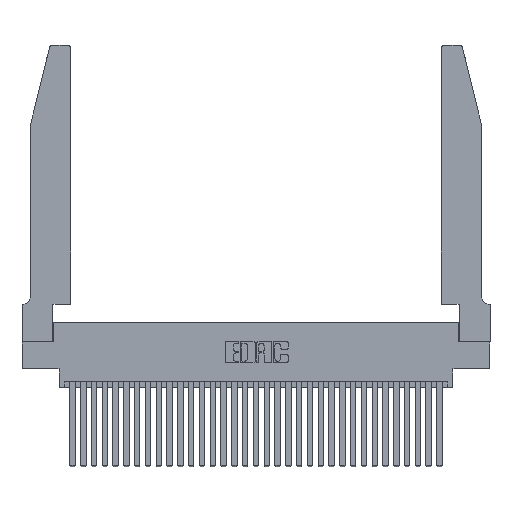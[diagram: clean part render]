
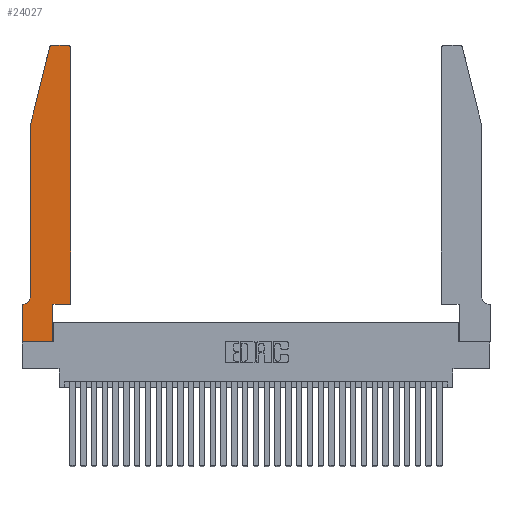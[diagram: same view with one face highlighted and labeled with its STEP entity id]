
A CAD part, top view. The second image highlights one B-rep face of the part: STEP entity #24027.
In plain terms, the highlighted planar face has unit normal (0, 0, 1).
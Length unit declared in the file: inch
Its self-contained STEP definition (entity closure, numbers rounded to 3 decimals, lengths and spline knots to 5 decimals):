
#411 = AXIS2_PLACEMENT_3D ( 'NONE', #13067, #10168, #25579 ) ;
#999 = CARTESIAN_POINT ( 'NONE',  ( 0.0755, 2., 0.37 ) ) ;
#1209 = CARTESIAN_POINT ( 'NONE',  ( 0.4505, 2.72, 0.37 ) ) ;
#1356 = LINE ( 'NONE', #23913, #9742 ) ;
#1509 = DIRECTION ( 'NONE',  ( -1., 0., 0. ) ) ;
#1685 = CARTESIAN_POINT ( 'NONE',  ( 0.2865, 0., 0.37 ) ) ;
#1832 = EDGE_CURVE ( 'NONE', #4338, #18854, #30496, .T. ) ;
#1875 = VERTEX_POINT ( 'NONE', #2177 ) ;
#1903 = LINE ( 'NONE', #19089, #4674 ) ;
#1988 = AXIS2_PLACEMENT_3D ( 'NONE', #17093, #2187, #29643 ) ;
#2177 = CARTESIAN_POINT ( 'NONE',  ( 0.284, 2.75, 0.37 ) ) ;
#2187 = DIRECTION ( 'NONE',  ( 0., 0., 1. ) ) ;
#2234 = LINE ( 'NONE', #25883, #6675 ) ;
#2886 = DIRECTION ( 'NONE',  ( 1., 0., 0. ) ) ;
#3325 = ORIENTED_EDGE ( 'NONE', *, *, #1832, .T. ) ;
#3663 = LINE ( 'NONE', #13820, #12471 ) ;
#3780 = DIRECTION ( 'NONE',  ( 0., -1., 0. ) ) ;
#3794 = ORIENTED_EDGE ( 'NONE', *, *, #19834, .T. ) ;
#4338 = VERTEX_POINT ( 'NONE', #27842 ) ;
#4674 = VECTOR ( 'NONE', #3780, 39.37008 ) ;
#5346 = PLANE ( 'NONE',  #411 ) ;
#5381 = VERTEX_POINT ( 'NONE', #8196 ) ;
#6237 = CIRCLE ( 'NONE', #1988, 0.03 ) ;
#6628 = FACE_OUTER_BOUND ( 'NONE', #9629, .T. ) ;
#6675 = VECTOR ( 'NONE', #2886, 39.37008 ) ;
#7281 = CIRCLE ( 'NONE', #28473, 0.03 ) ;
#7554 = DIRECTION ( 'NONE',  ( 0., 0., 1. ) ) ;
#7750 = ORIENTED_EDGE ( 'NONE', *, *, #16142, .T. ) ;
#8196 = CARTESIAN_POINT ( 'NONE',  ( 0.4205, 2.75, 0.37 ) ) ;
#8215 = ORIENTED_EDGE ( 'NONE', *, *, #14040, .T. ) ;
#8622 = ORIENTED_EDGE ( 'NONE', *, *, #14255, .T. ) ;
#9404 = CARTESIAN_POINT ( 'NONE',  ( 0., 0., 0.37 ) ) ;
#9629 = EDGE_LOOP ( 'NONE', ( #24375, #29802, #29660, #8622, #3325, #3794, #8215, #16254, #21913, #7750, #10709, #12995 ) ) ;
#9638 = VERTEX_POINT ( 'NONE', #17158 ) ;
#9742 = VECTOR ( 'NONE', #19107, 39.37008 ) ;
#10168 = DIRECTION ( 'NONE',  ( 0., 0., 1. ) ) ;
#10709 = ORIENTED_EDGE ( 'NONE', *, *, #17908, .T. ) ;
#12313 = AXIS2_PLACEMENT_3D ( 'NONE', #17534, #12477, #25004 ) ;
#12471 = VECTOR ( 'NONE', #29265, 39.37008 ) ;
#12477 = DIRECTION ( 'NONE',  ( 0., 0., -1. ) ) ;
#12713 = CARTESIAN_POINT ( 'NONE',  ( 0.2865, 0.35, 0.37 ) ) ;
#12995 = ORIENTED_EDGE ( 'NONE', *, *, #32623, .T. ) ;
#13067 = CARTESIAN_POINT ( 'NONE',  ( 0., 0.35, 0.37 ) ) ;
#13820 = CARTESIAN_POINT ( 'NONE',  ( 0.2605, 2.75, 0.37 ) ) ;
#14040 = EDGE_CURVE ( 'NONE', #9638, #29426, #1903, .T. ) ;
#14255 = EDGE_CURVE ( 'NONE', #29400, #4338, #18671, .T. ) ;
#14325 = DIRECTION ( 'NONE',  ( 1., 0., 0. ) ) ;
#14371 = VERTEX_POINT ( 'NONE', #19503 ) ;
#14756 = LINE ( 'NONE', #20382, #18322 ) ;
#14765 = CARTESIAN_POINT ( 'NONE',  ( 0.0755, 2., 0.37 ) ) ;
#15058 = EDGE_CURVE ( 'NONE', #1875, #17614, #6237, .T. ) ;
#15329 = LINE ( 'NONE', #24484, #25692 ) ;
#16114 = CARTESIAN_POINT ( 'NONE',  ( 0.4505, 0.35, 0.37 ) ) ;
#16142 = EDGE_CURVE ( 'NONE', #19496, #14371, #2234, .T. ) ;
#16254 = ORIENTED_EDGE ( 'NONE', *, *, #24840, .T. ) ;
#17093 = CARTESIAN_POINT ( 'NONE',  ( 0.284, 2.72, 0.37 ) ) ;
#17158 = CARTESIAN_POINT ( 'NONE',  ( 0., 0.35, 0.37 ) ) ;
#17427 = CARTESIAN_POINT ( 'NONE',  ( 0.4205, 2.72, 0.37 ) ) ;
#17497 = VECTOR ( 'NONE', #24241, 39.37008 ) ;
#17534 = CARTESIAN_POINT ( 'NONE',  ( 0.0055, 0.42, 0.37 ) ) ;
#17614 = VERTEX_POINT ( 'NONE', #29901 ) ;
#17908 = EDGE_CURVE ( 'NONE', #14371, #21235, #32936, .T. ) ;
#18322 = VECTOR ( 'NONE', #28211, 39.37008 ) ;
#18383 = DIRECTION ( 'NONE',  ( 0., 1., 0. ) ) ;
#18671 = LINE ( 'NONE', #999, #17497 ) ;
#18854 = VERTEX_POINT ( 'NONE', #30739 ) ;
#19089 = CARTESIAN_POINT ( 'NONE',  ( 0., 0., 0.37 ) ) ;
#19107 = DIRECTION ( 'NONE',  ( 0., 1., 0. ) ) ;
#19496 = VERTEX_POINT ( 'NONE', #12713 ) ;
#19503 = CARTESIAN_POINT ( 'NONE',  ( 0.4505, 0.35, 0.37 ) ) ;
#19834 = EDGE_CURVE ( 'NONE', #18854, #9638, #23213, .T. ) ;
#20352 = VERTEX_POINT ( 'NONE', #1685 ) ;
#20382 = CARTESIAN_POINT ( 'NONE',  ( 0.0755, 2., 0.37 ) ) ;
#21101 = EDGE_CURVE ( 'NONE', #17614, #29400, #14756, .T. ) ;
#21235 = VERTEX_POINT ( 'NONE', #1209 ) ;
#21913 = ORIENTED_EDGE ( 'NONE', *, *, #24751, .T. ) ;
#22615 = CARTESIAN_POINT ( 'NONE',  ( 0.0755, 0.35, 0.37 ) ) ;
#22852 = DIRECTION ( 'NONE',  ( 1., 0., 0. ) ) ;
#23213 = LINE ( 'NONE', #22615, #29267 ) ;
#23913 = CARTESIAN_POINT ( 'NONE',  ( 0.2865, 0.35, 0.37 ) ) ;
#24027 = ADVANCED_FACE ( 'NONE', ( #6628 ), #5346, .T. ) ;
#24241 = DIRECTION ( 'NONE',  ( 0., -1., 0. ) ) ;
#24375 = ORIENTED_EDGE ( 'NONE', *, *, #32944, .T. ) ;
#24484 = CARTESIAN_POINT ( 'NONE',  ( 0., 0., 0.37 ) ) ;
#24751 = EDGE_CURVE ( 'NONE', #20352, #19496, #1356, .T. ) ;
#24840 = EDGE_CURVE ( 'NONE', #29426, #20352, #15329, .T. ) ;
#25004 = DIRECTION ( 'NONE',  ( -1., 0., 0. ) ) ;
#25579 = DIRECTION ( 'NONE',  ( 1., 0., 0. ) ) ;
#25692 = VECTOR ( 'NONE', #14325, 39.37008 ) ;
#25883 = CARTESIAN_POINT ( 'NONE',  ( 0.4505, 0.35, 0.37 ) ) ;
#27842 = CARTESIAN_POINT ( 'NONE',  ( 0.0755, 0.42, 0.37 ) ) ;
#28211 = DIRECTION ( 'NONE',  ( -0.239, -0.971, 0. ) ) ;
#28473 = AXIS2_PLACEMENT_3D ( 'NONE', #17427, #7554, #22852 ) ;
#29265 = DIRECTION ( 'NONE',  ( -1., 0., 0. ) ) ;
#29267 = VECTOR ( 'NONE', #1509, 39.37008 ) ;
#29400 = VERTEX_POINT ( 'NONE', #14765 ) ;
#29426 = VERTEX_POINT ( 'NONE', #9404 ) ;
#29643 = DIRECTION ( 'NONE',  ( 1., 0., 0. ) ) ;
#29660 = ORIENTED_EDGE ( 'NONE', *, *, #21101, .T. ) ;
#29802 = ORIENTED_EDGE ( 'NONE', *, *, #15058, .T. ) ;
#29901 = CARTESIAN_POINT ( 'NONE',  ( 0.25487, 2.72718, 0.37 ) ) ;
#30496 = CIRCLE ( 'NONE', #12313, 0.07 ) ;
#30739 = CARTESIAN_POINT ( 'NONE',  ( 0.0055, 0.35, 0.37 ) ) ;
#30943 = VECTOR ( 'NONE', #18383, 39.37008 ) ;
#32623 = EDGE_CURVE ( 'NONE', #21235, #5381, #7281, .T. ) ;
#32936 = LINE ( 'NONE', #16114, #30943 ) ;
#32944 = EDGE_CURVE ( 'NONE', #5381, #1875, #3663, .T. ) ;
